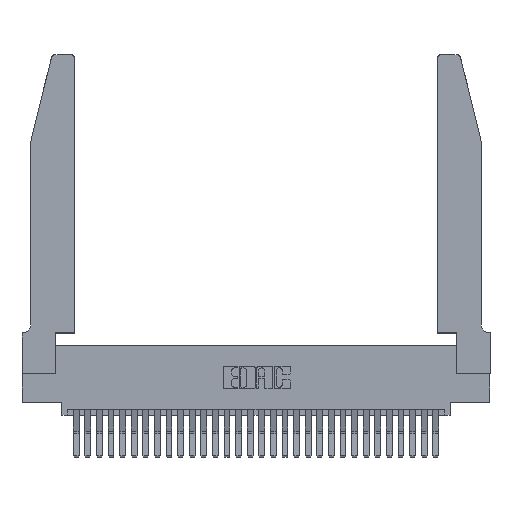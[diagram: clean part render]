
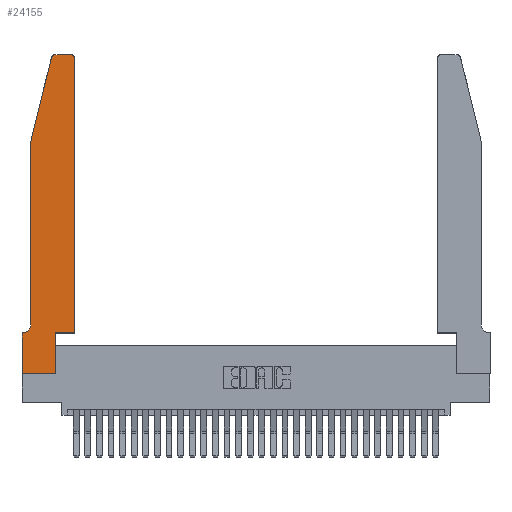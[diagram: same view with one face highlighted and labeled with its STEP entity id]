
A CAD part, top view. The second image highlights one B-rep face of the part: STEP entity #24155.
In plain terms, the highlighted planar face has unit normal (0, 0, 1).
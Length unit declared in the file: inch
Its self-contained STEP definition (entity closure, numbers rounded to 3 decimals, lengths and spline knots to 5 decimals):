
#68 = CARTESIAN_POINT ( 'NONE',  ( 0.0755, 2., 0.37 ) ) ;
#268 = VECTOR ( 'NONE', #13170, 39.37008 ) ;
#424 = ORIENTED_EDGE ( 'NONE', *, *, #22848, .T. ) ;
#1826 = VERTEX_POINT ( 'NONE', #68 ) ;
#2466 = CARTESIAN_POINT ( 'NONE',  ( 0.284, 2.72, 0.37 ) ) ;
#2833 = LINE ( 'NONE', #15326, #30888 ) ;
#2952 = CARTESIAN_POINT ( 'NONE',  ( 0., 0., 0.37 ) ) ;
#3008 = EDGE_CURVE ( 'NONE', #6623, #30329, #8174, .T. ) ;
#3632 = ORIENTED_EDGE ( 'NONE', *, *, #18673, .T. ) ;
#3778 = CARTESIAN_POINT ( 'NONE',  ( 0.4205, 2.75, 0.37 ) ) ;
#3915 = CARTESIAN_POINT ( 'NONE',  ( 0.2605, 2.75, 0.37 ) ) ;
#4889 = EDGE_CURVE ( 'NONE', #30329, #21155, #20143, .T. ) ;
#4961 = DIRECTION ( 'NONE',  ( 1., 0., 0. ) ) ;
#5105 = CARTESIAN_POINT ( 'NONE',  ( 0., 0., 0.37 ) ) ;
#5449 = DIRECTION ( 'NONE',  ( 1., 0., 0. ) ) ;
#5570 = CARTESIAN_POINT ( 'NONE',  ( 0.4505, 0.35, 0.37 ) ) ;
#5743 = VERTEX_POINT ( 'NONE', #3778 ) ;
#5812 = VECTOR ( 'NONE', #8230, 39.37008 ) ;
#6031 = CARTESIAN_POINT ( 'NONE',  ( 0.4505, 0.35, 0.37 ) ) ;
#6177 = CARTESIAN_POINT ( 'NONE',  ( 0.0055, 0.42, 0.37 ) ) ;
#6199 = LINE ( 'NONE', #6803, #19067 ) ;
#6415 = FACE_OUTER_BOUND ( 'NONE', #20791, .T. ) ;
#6499 = PLANE ( 'NONE',  #29831 ) ;
#6623 = VERTEX_POINT ( 'NONE', #10898 ) ;
#6803 = CARTESIAN_POINT ( 'NONE',  ( 0.0755, 0.35, 0.37 ) ) ;
#6806 = ORIENTED_EDGE ( 'NONE', *, *, #4889, .T. ) ;
#6840 = ORIENTED_EDGE ( 'NONE', *, *, #10753, .T. ) ;
#6877 = LINE ( 'NONE', #10758, #268 ) ;
#7137 = EDGE_CURVE ( 'NONE', #20674, #17399, #6877, .T. ) ;
#7215 = ORIENTED_EDGE ( 'NONE', *, *, #7137, .T. ) ;
#7305 = EDGE_CURVE ( 'NONE', #5743, #20063, #28439, .T. ) ;
#7308 = VECTOR ( 'NONE', #5449, 39.37008 ) ;
#8174 = LINE ( 'NONE', #26475, #25905 ) ;
#8230 = DIRECTION ( 'NONE',  ( 0., 1., 0. ) ) ;
#8589 = DIRECTION ( 'NONE',  ( 0., 1., 0. ) ) ;
#8619 = CARTESIAN_POINT ( 'NONE',  ( 0.2865, 0.35, 0.37 ) ) ;
#8626 = DIRECTION ( 'NONE',  ( -1., 0., 0. ) ) ;
#8954 = DIRECTION ( 'NONE',  ( 0., 0., 1. ) ) ;
#9971 = VECTOR ( 'NONE', #20962, 39.37008 ) ;
#10113 = LINE ( 'NONE', #6031, #28593 ) ;
#10751 = VERTEX_POINT ( 'NONE', #13348 ) ;
#10753 = EDGE_CURVE ( 'NONE', #17399, #10751, #10113, .T. ) ;
#10758 = CARTESIAN_POINT ( 'NONE',  ( 0.4505, 0.35, 0.37 ) ) ;
#10898 = CARTESIAN_POINT ( 'NONE',  ( 0., 0.35, 0.37 ) ) ;
#11067 = ORIENTED_EDGE ( 'NONE', *, *, #16328, .T. ) ;
#11372 = LINE ( 'NONE', #15437, #5812 ) ;
#11739 = EDGE_CURVE ( 'NONE', #12255, #1826, #2833, .T. ) ;
#12255 = VERTEX_POINT ( 'NONE', #14891 ) ;
#12792 = AXIS2_PLACEMENT_3D ( 'NONE', #2466, #19477, #4961 ) ;
#12927 = DIRECTION ( 'NONE',  ( 0., 0., 1. ) ) ;
#13170 = DIRECTION ( 'NONE',  ( 1., 0., 0. ) ) ;
#13348 = CARTESIAN_POINT ( 'NONE',  ( 0.4505, 2.72, 0.37 ) ) ;
#13567 = VERTEX_POINT ( 'NONE', #21575 ) ;
#14794 = ORIENTED_EDGE ( 'NONE', *, *, #26952, .T. ) ;
#14891 = CARTESIAN_POINT ( 'NONE',  ( 0.25487, 2.72718, 0.37 ) ) ;
#15326 = CARTESIAN_POINT ( 'NONE',  ( 0.0755, 2., 0.37 ) ) ;
#15437 = CARTESIAN_POINT ( 'NONE',  ( 0.2865, 0.35, 0.37 ) ) ;
#15764 = VERTEX_POINT ( 'NONE', #18039 ) ;
#16256 = CARTESIAN_POINT ( 'NONE',  ( 0.0755, 2., 0.37 ) ) ;
#16272 = CARTESIAN_POINT ( 'NONE',  ( 0.284, 2.75, 0.37 ) ) ;
#16328 = EDGE_CURVE ( 'NONE', #10751, #5743, #16624, .T. ) ;
#16624 = CIRCLE ( 'NONE', #18989, 0.03 ) ;
#17399 = VERTEX_POINT ( 'NONE', #5570 ) ;
#18039 = CARTESIAN_POINT ( 'NONE',  ( 0.0055, 0.35, 0.37 ) ) ;
#18658 = DIRECTION ( 'NONE',  ( 0., -1., 0. ) ) ;
#18673 = EDGE_CURVE ( 'NONE', #13567, #15764, #24096, .T. ) ;
#18989 = AXIS2_PLACEMENT_3D ( 'NONE', #27380, #12927, #29808 ) ;
#19067 = VECTOR ( 'NONE', #21258, 39.37008 ) ;
#19477 = DIRECTION ( 'NONE',  ( 0., 0., 1. ) ) ;
#20063 = VERTEX_POINT ( 'NONE', #16272 ) ;
#20143 = LINE ( 'NONE', #2952, #7308 ) ;
#20674 = VERTEX_POINT ( 'NONE', #8619 ) ;
#20791 = EDGE_LOOP ( 'NONE', ( #29953, #28855, #20930, #424, #3632, #28189, #27055, #6806, #14794, #7215, #6840, #11067 ) ) ;
#20930 = ORIENTED_EDGE ( 'NONE', *, *, #11739, .T. ) ;
#20962 = DIRECTION ( 'NONE',  ( -1., 0., 0. ) ) ;
#20963 = CARTESIAN_POINT ( 'NONE',  ( 0., 0.35, 0.37 ) ) ;
#21155 = VERTEX_POINT ( 'NONE', #31306 ) ;
#21258 = DIRECTION ( 'NONE',  ( -1., 0., 0. ) ) ;
#21575 = CARTESIAN_POINT ( 'NONE',  ( 0.0755, 0.42, 0.37 ) ) ;
#21597 = EDGE_CURVE ( 'NONE', #15764, #6623, #6199, .T. ) ;
#22540 = DIRECTION ( 'NONE',  ( -0.239, -0.971, 0. ) ) ;
#22736 = VECTOR ( 'NONE', #18658, 39.37008 ) ;
#22839 = AXIS2_PLACEMENT_3D ( 'NONE', #6177, #23058, #8626 ) ;
#22848 = EDGE_CURVE ( 'NONE', #1826, #13567, #24257, .T. ) ;
#23058 = DIRECTION ( 'NONE',  ( 0., 0., -1. ) ) ;
#24096 = CIRCLE ( 'NONE', #22839, 0.07 ) ;
#24155 = ADVANCED_FACE ( 'NONE', ( #6415 ), #6499, .T. ) ;
#24257 = LINE ( 'NONE', #16256, #22736 ) ;
#25189 = CIRCLE ( 'NONE', #12792, 0.03 ) ;
#25814 = DIRECTION ( 'NONE',  ( 1., 0., 0. ) ) ;
#25905 = VECTOR ( 'NONE', #31332, 39.37008 ) ;
#26475 = CARTESIAN_POINT ( 'NONE',  ( 0., 0., 0.37 ) ) ;
#26952 = EDGE_CURVE ( 'NONE', #21155, #20674, #11372, .T. ) ;
#27055 = ORIENTED_EDGE ( 'NONE', *, *, #3008, .T. ) ;
#27380 = CARTESIAN_POINT ( 'NONE',  ( 0.4205, 2.72, 0.37 ) ) ;
#28189 = ORIENTED_EDGE ( 'NONE', *, *, #21597, .T. ) ;
#28439 = LINE ( 'NONE', #3915, #9971 ) ;
#28593 = VECTOR ( 'NONE', #8589, 39.37008 ) ;
#28855 = ORIENTED_EDGE ( 'NONE', *, *, #30878, .T. ) ;
#29808 = DIRECTION ( 'NONE',  ( 1., 0., 0. ) ) ;
#29831 = AXIS2_PLACEMENT_3D ( 'NONE', #20963, #8954, #25814 ) ;
#29953 = ORIENTED_EDGE ( 'NONE', *, *, #7305, .T. ) ;
#30329 = VERTEX_POINT ( 'NONE', #5105 ) ;
#30878 = EDGE_CURVE ( 'NONE', #20063, #12255, #25189, .T. ) ;
#30888 = VECTOR ( 'NONE', #22540, 39.37008 ) ;
#31306 = CARTESIAN_POINT ( 'NONE',  ( 0.2865, 0., 0.37 ) ) ;
#31332 = DIRECTION ( 'NONE',  ( 0., -1., 0. ) ) ;
